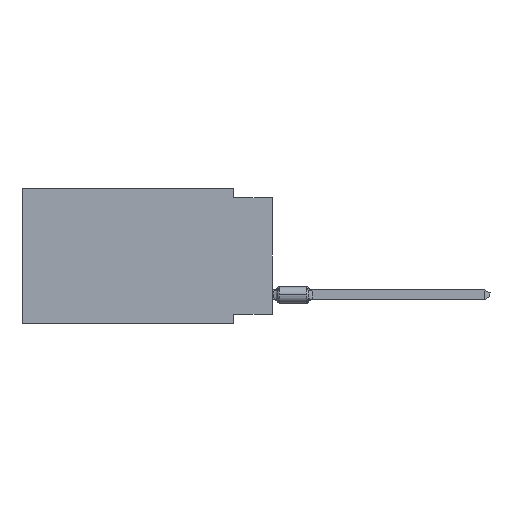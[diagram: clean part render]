
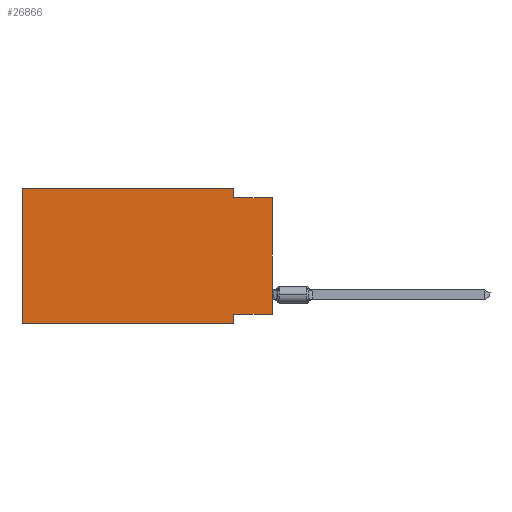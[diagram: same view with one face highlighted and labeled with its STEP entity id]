
A CAD part, left-side view. The second image highlights one B-rep face of the part: STEP entity #26866.
In plain terms, the highlighted planar face has unit normal (-1, 0, 0).
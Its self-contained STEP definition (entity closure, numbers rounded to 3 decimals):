
#190 = EDGE_CURVE ( 'NONE', #40845, #7943, #22602, .T. ) ;
#1186 = DIRECTION ( 'NONE',  ( 0., 0., -1. ) ) ;
#2021 = EDGE_CURVE ( 'NONE', #44116, #4734, #42493, .T. ) ;
#2053 = CARTESIAN_POINT ( 'NONE',  ( 0., 0., -0.635 ) ) ;
#2964 = EDGE_CURVE ( 'NONE', #9592, #7771, #27311, .T. ) ;
#4734 = VERTEX_POINT ( 'NONE', #9532 ) ;
#5677 = FACE_OUTER_BOUND ( 'NONE', #24378, .T. ) ;
#6459 = VECTOR ( 'NONE', #49296, 1000. ) ;
#6873 = CARTESIAN_POINT ( 'NONE',  ( 0., 0., 0. ) ) ;
#7771 = VERTEX_POINT ( 'NONE', #2053 ) ;
#7943 = VERTEX_POINT ( 'NONE', #34660 ) ;
#9532 = CARTESIAN_POINT ( 'NONE',  ( 0., 2.54, -8.255 ) ) ;
#9592 = VERTEX_POINT ( 'NONE', #21513 ) ;
#10271 = ORIENTED_EDGE ( 'NONE', *, *, #20661, .F. ) ;
#13849 = VECTOR ( 'NONE', #15067, 1000. ) ;
#14212 = LINE ( 'NONE', #44826, #20478 ) ;
#14376 = CARTESIAN_POINT ( 'NONE',  ( 0., 2.54, 0. ) ) ;
#14404 = LINE ( 'NONE', #6873, #28157 ) ;
#15067 = DIRECTION ( 'NONE',  ( 0., 0., 1. ) ) ;
#15278 = CARTESIAN_POINT ( 'NONE',  ( 0., 0., -0.635 ) ) ;
#15469 = CARTESIAN_POINT ( 'NONE',  ( 0., 2.54, 0. ) ) ;
#15621 = ORIENTED_EDGE ( 'NONE', *, *, #41929, .T. ) ;
#16563 = VECTOR ( 'NONE', #19762, 1000. ) ;
#18228 = DIRECTION ( 'NONE',  ( 0., -1., 0. ) ) ;
#19523 = EDGE_CURVE ( 'NONE', #40845, #23857, #14212, .T. ) ;
#19672 = CARTESIAN_POINT ( 'NONE',  ( 0., 0., -8.255 ) ) ;
#19762 = DIRECTION ( 'NONE',  ( 0., 0., -1. ) ) ;
#20478 = VECTOR ( 'NONE', #18228, 1000. ) ;
#20661 = EDGE_CURVE ( 'NONE', #4734, #23857, #31293, .T. ) ;
#21513 = CARTESIAN_POINT ( 'NONE',  ( 0., 2.54, -0.635 ) ) ;
#22602 = LINE ( 'NONE', #37896, #13849 ) ;
#23266 = CARTESIAN_POINT ( 'NONE',  ( 0., 2.54, -8.89 ) ) ;
#23857 = VERTEX_POINT ( 'NONE', #28446 ) ;
#23990 = VECTOR ( 'NONE', #35055, 1000. ) ;
#24378 = EDGE_LOOP ( 'NONE', ( #15621, #34378, #30060, #31651, #29383, #30649, #10271, #38153 ) ) ;
#24787 = CARTESIAN_POINT ( 'NONE',  ( 0., 0., -8.255 ) ) ;
#26866 = ADVANCED_FACE ( 'NONE', ( #5677 ), #36321, .F. ) ;
#27311 = LINE ( 'NONE', #15278, #45365 ) ;
#27403 = VERTEX_POINT ( 'NONE', #14376 ) ;
#28157 = VECTOR ( 'NONE', #47811, 1000. ) ;
#28446 = CARTESIAN_POINT ( 'NONE',  ( 0., 2.54, -8.89 ) ) ;
#29383 = ORIENTED_EDGE ( 'NONE', *, *, #190, .F. ) ;
#30060 = ORIENTED_EDGE ( 'NONE', *, *, #33517, .F. ) ;
#30586 = DIRECTION ( 'NONE',  ( 0., -1., 0. ) ) ;
#30649 = ORIENTED_EDGE ( 'NONE', *, *, #19523, .T. ) ;
#31293 = LINE ( 'NONE', #23266, #16563 ) ;
#31651 = ORIENTED_EDGE ( 'NONE', *, *, #42000, .F. ) ;
#33517 = EDGE_CURVE ( 'NONE', #27403, #9592, #49625, .T. ) ;
#33964 = CARTESIAN_POINT ( 'NONE',  ( 0., 16.383, 0. ) ) ;
#34223 = LINE ( 'NONE', #33964, #6459 ) ;
#34234 = DIRECTION ( 'NONE',  ( 0., 1., 0. ) ) ;
#34378 = ORIENTED_EDGE ( 'NONE', *, *, #2964, .F. ) ;
#34660 = CARTESIAN_POINT ( 'NONE',  ( 0., 16.383, 0. ) ) ;
#35055 = DIRECTION ( 'NONE',  ( 0., 0., -1. ) ) ;
#36321 = PLANE ( 'NONE',  #38845 ) ;
#36342 = CARTESIAN_POINT ( 'NONE',  ( 0., 16.383, -8.89 ) ) ;
#37896 = CARTESIAN_POINT ( 'NONE',  ( 0., 16.383, 0. ) ) ;
#38153 = ORIENTED_EDGE ( 'NONE', *, *, #2021, .F. ) ;
#38845 = AXIS2_PLACEMENT_3D ( 'NONE', #39588, #47142, #1186 ) ;
#39588 = CARTESIAN_POINT ( 'NONE',  ( 0., 16.383, 0. ) ) ;
#40845 = VERTEX_POINT ( 'NONE', #36342 ) ;
#41929 = EDGE_CURVE ( 'NONE', #44116, #7771, #14404, .T. ) ;
#42000 = EDGE_CURVE ( 'NONE', #7943, #27403, #34223, .T. ) ;
#42493 = LINE ( 'NONE', #19672, #47671 ) ;
#44116 = VERTEX_POINT ( 'NONE', #24787 ) ;
#44826 = CARTESIAN_POINT ( 'NONE',  ( 0., 16.383, -8.89 ) ) ;
#45365 = VECTOR ( 'NONE', #30586, 1000. ) ;
#47142 = DIRECTION ( 'NONE',  ( 1., 0., 0. ) ) ;
#47671 = VECTOR ( 'NONE', #34234, 1000. ) ;
#47811 = DIRECTION ( 'NONE',  ( 0., 0., 1. ) ) ;
#49296 = DIRECTION ( 'NONE',  ( 0., -1., 0. ) ) ;
#49625 = LINE ( 'NONE', #15469, #23990 ) ;
